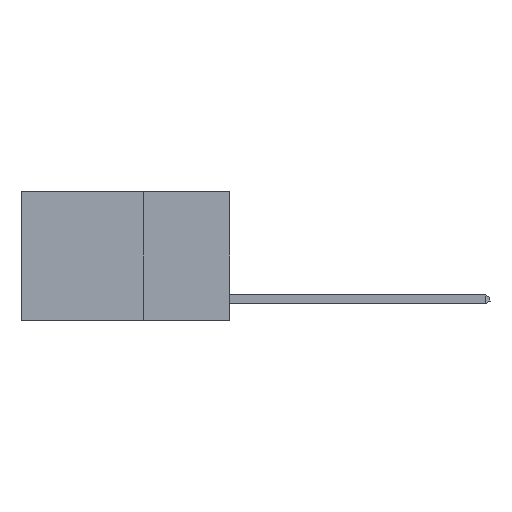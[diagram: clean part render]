
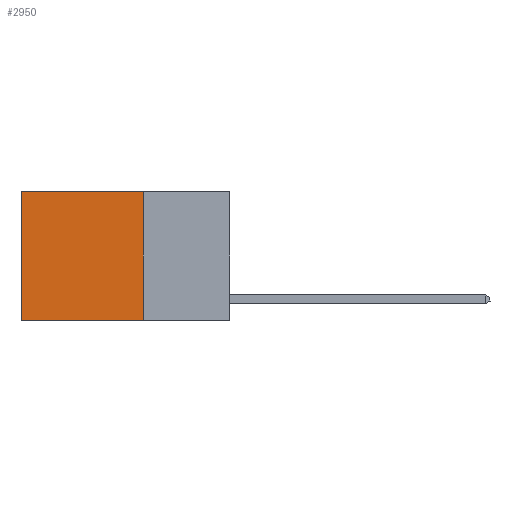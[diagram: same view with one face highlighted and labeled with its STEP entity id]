
A CAD part, left-side view. The second image highlights one B-rep face of the part: STEP entity #2950.
In plain terms, the highlighted planar face has unit normal (-1, 0, 0).
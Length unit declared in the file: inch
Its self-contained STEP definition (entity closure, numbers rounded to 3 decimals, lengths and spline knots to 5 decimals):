
#1682 = DIRECTION ( 'NONE',  ( 0., 0., -1. ) ) ;
#1955 = ORIENTED_EDGE ( 'NONE', *, *, #2474, .F. ) ;
#2222 = DIRECTION ( 'NONE',  ( 0., 0., -1. ) ) ;
#2474 = EDGE_CURVE ( 'NONE', #16437, #9147, #11046, .T. ) ;
#2620 = FACE_OUTER_BOUND ( 'NONE', #8288, .T. ) ;
#2950 = ADVANCED_FACE ( 'NONE', ( #2620 ), #7216, .F. ) ;
#3016 = CARTESIAN_POINT ( 'NONE',  ( 0.2625, 0.25, -0.37 ) ) ;
#3239 = DIRECTION ( 'NONE',  ( 0., 1., 0. ) ) ;
#3398 = DIRECTION ( 'NONE',  ( 0., 1., 0. ) ) ;
#3408 = VECTOR ( 'NONE', #3398, 39.37008 ) ;
#4805 = ORIENTED_EDGE ( 'NONE', *, *, #14947, .F. ) ;
#4857 = DIRECTION ( 'NONE',  ( 0., 0., -1. ) ) ;
#4989 = CARTESIAN_POINT ( 'NONE',  ( 0.2625, 0.6, 0. ) ) ;
#5878 = CARTESIAN_POINT ( 'NONE',  ( 0.2625, 0.25, 0. ) ) ;
#6468 = CARTESIAN_POINT ( 'NONE',  ( 0.2625, 0.25, 0. ) ) ;
#6652 = CARTESIAN_POINT ( 'NONE',  ( 0.2625, 0.6, 0. ) ) ;
#6654 = VECTOR ( 'NONE', #1682, 39.37008 ) ;
#7149 = ORIENTED_EDGE ( 'NONE', *, *, #8136, .T. ) ;
#7216 = PLANE ( 'NONE',  #8651 ) ;
#7225 = CARTESIAN_POINT ( 'NONE',  ( 0.2625, 0.25, -0.37 ) ) ;
#7424 = VECTOR ( 'NONE', #3239, 39.37008 ) ;
#8026 = EDGE_CURVE ( 'NONE', #12224, #9816, #14438, .T. ) ;
#8136 = EDGE_CURVE ( 'NONE', #9816, #9147, #13802, .T. ) ;
#8288 = EDGE_LOOP ( 'NONE', ( #7149, #1955, #4805, #17571 ) ) ;
#8651 = AXIS2_PLACEMENT_3D ( 'NONE', #5878, #10464, #2222 ) ;
#9147 = VERTEX_POINT ( 'NONE', #15386 ) ;
#9816 = VERTEX_POINT ( 'NONE', #6652 ) ;
#10464 = DIRECTION ( 'NONE',  ( 1., 0., 0. ) ) ;
#11046 = LINE ( 'NONE', #7225, #7424 ) ;
#11595 = VECTOR ( 'NONE', #4857, 39.37008 ) ;
#12224 = VERTEX_POINT ( 'NONE', #6468 ) ;
#13802 = LINE ( 'NONE', #4989, #11595 ) ;
#14438 = LINE ( 'NONE', #15740, #3408 ) ;
#14947 = EDGE_CURVE ( 'NONE', #12224, #16437, #17632, .T. ) ;
#15386 = CARTESIAN_POINT ( 'NONE',  ( 0.2625, 0.6, -0.37 ) ) ;
#15602 = CARTESIAN_POINT ( 'NONE',  ( 0.2625, 0.25, 0. ) ) ;
#15740 = CARTESIAN_POINT ( 'NONE',  ( 0.2625, 0.25, 0. ) ) ;
#16437 = VERTEX_POINT ( 'NONE', #3016 ) ;
#17571 = ORIENTED_EDGE ( 'NONE', *, *, #8026, .T. ) ;
#17632 = LINE ( 'NONE', #15602, #6654 ) ;
